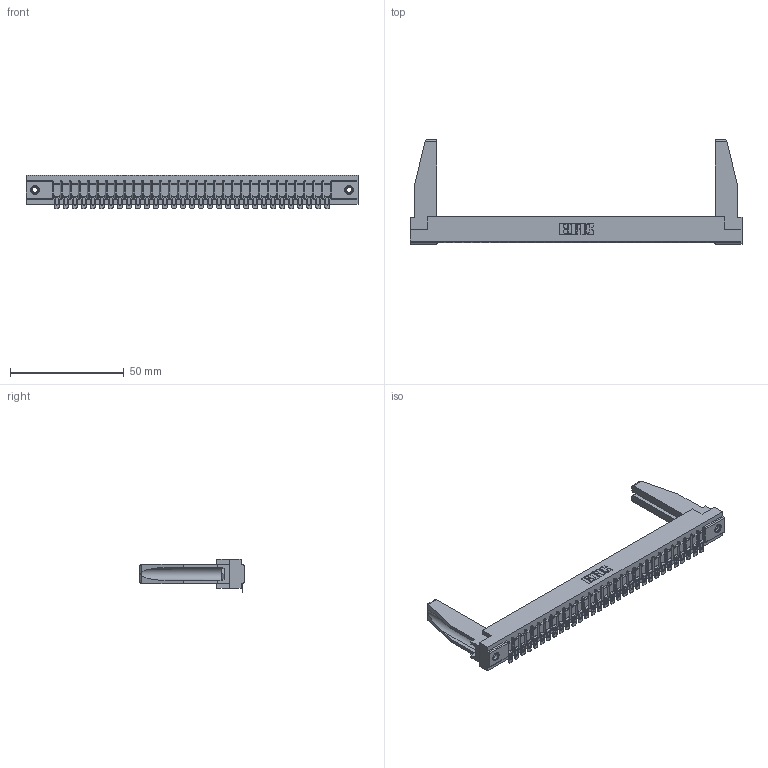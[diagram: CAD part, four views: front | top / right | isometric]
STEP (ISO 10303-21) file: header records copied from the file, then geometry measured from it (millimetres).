
FILE_DESCRIPTION (( 'STEP AP203' ), '1' );
FILE_NAME ('307-031-554-178.STEP', '2019-09-05T05:01:35', ( '' ), ( '' ), 'SwSTEP 2.0', 'SolidWorks 2016', '' );
FILE_SCHEMA (( 'CONFIG_CONTROL_DESIGN' ));
Length unit declared in the file: inch
Products named in the file (5): 307-031-554-178; 307 Part_.156 Dia Mounting Holes; 345-250-001_345-250-001-102; 307-290-002_554; 307-220-078
Assembly tree (36 placements, depth 2):
  307-031-554-178
    307 Part_.156 Dia Mounting Holes
    307-290-002_554  x31
    307-220-078  x2
    345-250-001_345-250-001-102  x2
Bounding box: 145.85 x 45.72 x 14.52 mm (x, y, z)
Volume: 19529.9 mm3; surface area: 23239 mm2
Topology: 36 solids, 36 shells, 2791 faces, 8496 edges, 5568 vertices
Faces by surface type: plane 1580, cylinder 1131, sphere 64, cone 12, torus 4
Entity records: 31336 total; most frequent: CARTESIAN_POINT 5284, ORIENTED_EDGE 5230, DIRECTION 5101, EDGE_CURVE 2615, LINE 1995, VECTOR 1995, VERTEX_POINT 1694, AXIS2_PLACEMENT_3D 1553
